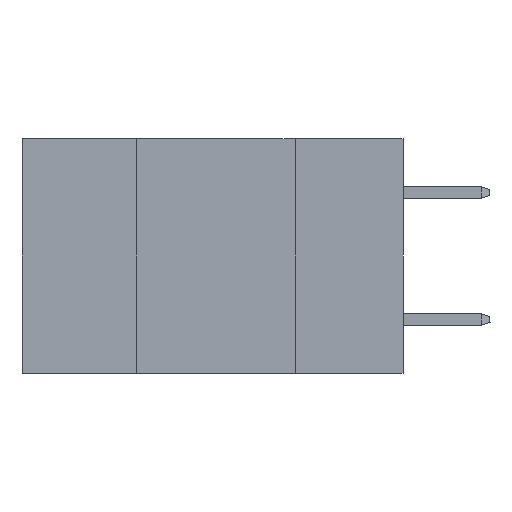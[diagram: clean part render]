
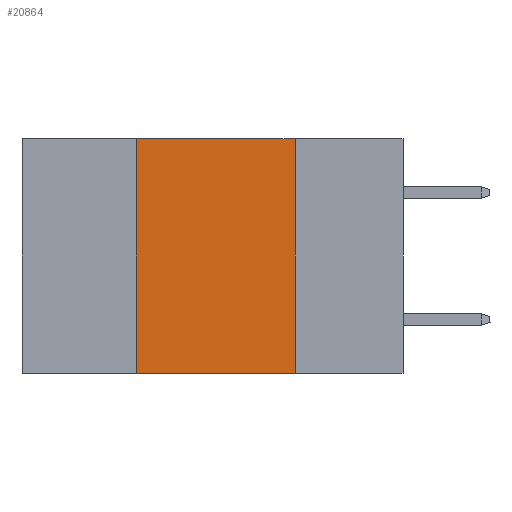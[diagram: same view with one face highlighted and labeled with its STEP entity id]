
A CAD part, left-side view. The second image highlights one B-rep face of the part: STEP entity #20864.
In plain terms, the highlighted planar face has unit normal (-1, 0, 0).
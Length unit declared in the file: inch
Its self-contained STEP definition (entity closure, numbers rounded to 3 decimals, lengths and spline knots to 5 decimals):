
#1154 = LINE ( 'NONE', #18793, #5144 ) ;
#1969 = EDGE_CURVE ( 'NONE', #11078, #15301, #9011, .T. ) ;
#2516 = VERTEX_POINT ( 'NONE', #20679 ) ;
#4102 = CARTESIAN_POINT ( 'NONE',  ( 0., 0.6, 0. ) ) ;
#5144 = VECTOR ( 'NONE', #5337, 39.37008 ) ;
#5317 = ORIENTED_EDGE ( 'NONE', *, *, #24508, .F. ) ;
#5337 = DIRECTION ( 'NONE',  ( 0., 0., 1. ) ) ;
#5874 = FACE_OUTER_BOUND ( 'NONE', #21389, .T. ) ;
#6644 = DIRECTION ( 'NONE',  ( 0., -1., 0. ) ) ;
#7135 = CARTESIAN_POINT ( 'NONE',  ( 0., 0.42, -0.37 ) ) ;
#7955 = VECTOR ( 'NONE', #8095, 39.37008 ) ;
#8095 = DIRECTION ( 'NONE',  ( 0., -1., 0. ) ) ;
#8114 = CARTESIAN_POINT ( 'NONE',  ( 0., 0.17, 0. ) ) ;
#8337 = VECTOR ( 'NONE', #9276, 39.37008 ) ;
#8773 = VERTEX_POINT ( 'NONE', #7135 ) ;
#9011 = LINE ( 'NONE', #24910, #8337 ) ;
#9276 = DIRECTION ( 'NONE',  ( 0., 0., -1. ) ) ;
#11078 = VERTEX_POINT ( 'NONE', #8114 ) ;
#11635 = DIRECTION ( 'NONE',  ( 0., 0., -1. ) ) ;
#11915 = EDGE_CURVE ( 'NONE', #8773, #15301, #14953, .T. ) ;
#12541 = ORIENTED_EDGE ( 'NONE', *, *, #13113, .F. ) ;
#13113 = EDGE_CURVE ( 'NONE', #8773, #2516, #1154, .T. ) ;
#14500 = LINE ( 'NONE', #20463, #21147 ) ;
#14953 = LINE ( 'NONE', #17616, #7955 ) ;
#15301 = VERTEX_POINT ( 'NONE', #20607 ) ;
#17616 = CARTESIAN_POINT ( 'NONE',  ( 0., 0.6, -0.37 ) ) ;
#18300 = ORIENTED_EDGE ( 'NONE', *, *, #11915, .T. ) ;
#18793 = CARTESIAN_POINT ( 'NONE',  ( 0., 0.42, 0. ) ) ;
#20463 = CARTESIAN_POINT ( 'NONE',  ( 0., 0.6, 0. ) ) ;
#20607 = CARTESIAN_POINT ( 'NONE',  ( 0., 0.17, -0.37 ) ) ;
#20679 = CARTESIAN_POINT ( 'NONE',  ( 0., 0.42, 0. ) ) ;
#20864 = ADVANCED_FACE ( 'NONE', ( #5874 ), #21615, .F. ) ;
#21076 = AXIS2_PLACEMENT_3D ( 'NONE', #4102, #21358, #11635 ) ;
#21147 = VECTOR ( 'NONE', #6644, 39.37008 ) ;
#21358 = DIRECTION ( 'NONE',  ( 1., 0., 0. ) ) ;
#21389 = EDGE_LOOP ( 'NONE', ( #21560, #5317, #12541, #18300 ) ) ;
#21560 = ORIENTED_EDGE ( 'NONE', *, *, #1969, .F. ) ;
#21615 = PLANE ( 'NONE',  #21076 ) ;
#24508 = EDGE_CURVE ( 'NONE', #2516, #11078, #14500, .T. ) ;
#24910 = CARTESIAN_POINT ( 'NONE',  ( 0., 0.17, 0. ) ) ;
